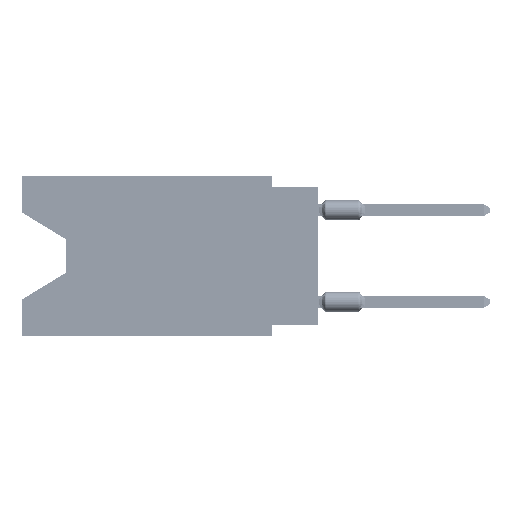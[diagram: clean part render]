
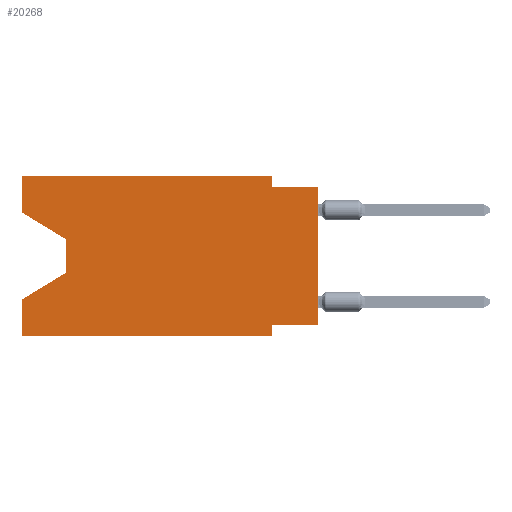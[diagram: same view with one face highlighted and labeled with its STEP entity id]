
A CAD part, left-side view. The second image highlights one B-rep face of the part: STEP entity #20268.
In plain terms, the highlighted planar face has unit normal (-1, 0, 0).
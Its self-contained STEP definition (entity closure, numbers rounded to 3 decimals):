
#35 = VECTOR ( 'NONE', #18206, 1000. ) ;
#1812 = ORIENTED_EDGE ( 'NONE', *, *, #26979, .F. ) ;
#2176 = LINE ( 'NONE', #37560, #27442 ) ;
#2943 = DIRECTION ( 'NONE',  ( 0., 1., 0. ) ) ;
#2965 = ORIENTED_EDGE ( 'NONE', *, *, #28584, .F. ) ;
#3649 = ORIENTED_EDGE ( 'NONE', *, *, #36116, .T. ) ;
#5922 = VERTEX_POINT ( 'NONE', #71807 ) ;
#6380 = VECTOR ( 'NONE', #44592, 1000. ) ;
#7038 = ORIENTED_EDGE ( 'NONE', *, *, #61734, .T. ) ;
#7966 = CARTESIAN_POINT ( 'NONE',  ( 0., 2.54, -8.89 ) ) ;
#8591 = CARTESIAN_POINT ( 'NONE',  ( 0., 16.383, 0. ) ) ;
#8744 = VERTEX_POINT ( 'NONE', #57537 ) ;
#9004 = EDGE_CURVE ( 'NONE', #44556, #27922, #29869, .T. ) ;
#9166 = DIRECTION ( 'NONE',  ( 0., -1., 0. ) ) ;
#9550 = LINE ( 'NONE', #32517, #25673 ) ;
#9578 = VERTEX_POINT ( 'NONE', #7966 ) ;
#12994 = LINE ( 'NONE', #37083, #18165 ) ;
#14210 = EDGE_CURVE ( 'NONE', #54224, #9578, #33137, .T. ) ;
#15890 = AXIS2_PLACEMENT_3D ( 'NONE', #19984, #43703, #32421 ) ;
#17105 = CARTESIAN_POINT ( 'NONE',  ( 0., 13.97, -3.505 ) ) ;
#18165 = VECTOR ( 'NONE', #60837, 1000. ) ;
#18206 = DIRECTION ( 'NONE',  ( 0., 0., 1. ) ) ;
#18877 = EDGE_CURVE ( 'NONE', #28221, #70979, #35831, .T. ) ;
#19884 = EDGE_CURVE ( 'NONE', #70979, #8744, #37947, .T. ) ;
#19984 = CARTESIAN_POINT ( 'NONE',  ( 0., 16.383, 0. ) ) ;
#20201 = EDGE_CURVE ( 'NONE', #27922, #28221, #35183, .T. ) ;
#20268 = ADVANCED_FACE ( 'NONE', ( #55393 ), #56157, .F. ) ;
#20823 = LINE ( 'NONE', #55856, #72713 ) ;
#23395 = VERTEX_POINT ( 'NONE', #60676 ) ;
#24446 = VECTOR ( 'NONE', #72033, 1000. ) ;
#24466 = DIRECTION ( 'NONE',  ( 0., 0.855, -0.519 ) ) ;
#24765 = CARTESIAN_POINT ( 'NONE',  ( 0., 2.54, 0. ) ) ;
#25241 = EDGE_LOOP ( 'NONE', ( #30478, #45612, #25558, #2965, #7038, #35270, #1812, #3649, #56038, #54397, #64348, #45249 ) ) ;
#25558 = ORIENTED_EDGE ( 'NONE', *, *, #73680, .T. ) ;
#25673 = VECTOR ( 'NONE', #57395, 1000. ) ;
#26979 = EDGE_CURVE ( 'NONE', #5922, #54224, #20823, .T. ) ;
#27442 = VECTOR ( 'NONE', #54706, 1000. ) ;
#27922 = VERTEX_POINT ( 'NONE', #8591 ) ;
#28221 = VERTEX_POINT ( 'NONE', #24765 ) ;
#28584 = EDGE_CURVE ( 'NONE', #55753, #42549, #12994, .T. ) ;
#29869 = LINE ( 'NONE', #36463, #35 ) ;
#30112 = CARTESIAN_POINT ( 'NONE',  ( 0., 16.383, -2.038 ) ) ;
#30478 = ORIENTED_EDGE ( 'NONE', *, *, #62757, .T. ) ;
#32421 = DIRECTION ( 'NONE',  ( 0., 0., -1. ) ) ;
#32517 = CARTESIAN_POINT ( 'NONE',  ( 0., 13.97, -3.505 ) ) ;
#33137 = LINE ( 'NONE', #56873, #39902 ) ;
#34991 = CARTESIAN_POINT ( 'NONE',  ( 0., 0., 0. ) ) ;
#35183 = LINE ( 'NONE', #53463, #54441 ) ;
#35270 = ORIENTED_EDGE ( 'NONE', *, *, #14210, .F. ) ;
#35279 = CARTESIAN_POINT ( 'NONE',  ( 0., 2.54, -8.255 ) ) ;
#35831 = LINE ( 'NONE', #48288, #24446 ) ;
#36116 = EDGE_CURVE ( 'NONE', #5922, #8744, #59117, .T. ) ;
#36463 = CARTESIAN_POINT ( 'NONE',  ( 0., 16.383, 0. ) ) ;
#37083 = CARTESIAN_POINT ( 'NONE',  ( 0., 16.383, 0. ) ) ;
#37560 = CARTESIAN_POINT ( 'NONE',  ( 0., 16.383, -8.89 ) ) ;
#37947 = LINE ( 'NONE', #72623, #64324 ) ;
#39902 = VECTOR ( 'NONE', #44432, 1000. ) ;
#41163 = VECTOR ( 'NONE', #71950, 1000. ) ;
#41974 = CARTESIAN_POINT ( 'NONE',  ( 0., 16.383, -6.852 ) ) ;
#42549 = VERTEX_POINT ( 'NONE', #41974 ) ;
#42808 = CARTESIAN_POINT ( 'NONE',  ( 0., 16.383, -8.89 ) ) ;
#43703 = DIRECTION ( 'NONE',  ( 1., 0., 0. ) ) ;
#43832 = LINE ( 'NONE', #67576, #6380 ) ;
#43899 = CARTESIAN_POINT ( 'NONE',  ( 0., 13.97, -5.385 ) ) ;
#44432 = DIRECTION ( 'NONE',  ( 0., 0., -1. ) ) ;
#44556 = VERTEX_POINT ( 'NONE', #30112 ) ;
#44592 = DIRECTION ( 'NONE',  ( 0., -0.855, -0.519 ) ) ;
#45249 = ORIENTED_EDGE ( 'NONE', *, *, #9004, .F. ) ;
#45612 = ORIENTED_EDGE ( 'NONE', *, *, #75224, .T. ) ;
#45865 = CARTESIAN_POINT ( 'NONE',  ( 0., 2.54, -0.635 ) ) ;
#46859 = DIRECTION ( 'NONE',  ( 0., -1., 0. ) ) ;
#48288 = CARTESIAN_POINT ( 'NONE',  ( 0., 2.54, 0. ) ) ;
#50524 = VECTOR ( 'NONE', #24466, 1000. ) ;
#53463 = CARTESIAN_POINT ( 'NONE',  ( 0., 16.383, 0. ) ) ;
#54034 = LINE ( 'NONE', #43899, #50524 ) ;
#54224 = VERTEX_POINT ( 'NONE', #35279 ) ;
#54397 = ORIENTED_EDGE ( 'NONE', *, *, #18877, .F. ) ;
#54441 = VECTOR ( 'NONE', #46859, 1000. ) ;
#54706 = DIRECTION ( 'NONE',  ( 0., -1., 0. ) ) ;
#55393 = FACE_OUTER_BOUND ( 'NONE', #25241, .T. ) ;
#55753 = VERTEX_POINT ( 'NONE', #42808 ) ;
#55856 = CARTESIAN_POINT ( 'NONE',  ( 0., 0., -8.255 ) ) ;
#56038 = ORIENTED_EDGE ( 'NONE', *, *, #19884, .F. ) ;
#56157 = PLANE ( 'NONE',  #15890 ) ;
#56873 = CARTESIAN_POINT ( 'NONE',  ( 0., 2.54, -8.89 ) ) ;
#57395 = DIRECTION ( 'NONE',  ( 0., 0., -1. ) ) ;
#57449 = VERTEX_POINT ( 'NONE', #17105 ) ;
#57537 = CARTESIAN_POINT ( 'NONE',  ( 0., 0., -0.635 ) ) ;
#59117 = LINE ( 'NONE', #34991, #41163 ) ;
#60676 = CARTESIAN_POINT ( 'NONE',  ( 0., 13.97, -5.385 ) ) ;
#60837 = DIRECTION ( 'NONE',  ( 0., 0., 1. ) ) ;
#61734 = EDGE_CURVE ( 'NONE', #55753, #9578, #2176, .T. ) ;
#62757 = EDGE_CURVE ( 'NONE', #44556, #57449, #43832, .T. ) ;
#64324 = VECTOR ( 'NONE', #9166, 1000. ) ;
#64348 = ORIENTED_EDGE ( 'NONE', *, *, #20201, .F. ) ;
#67576 = CARTESIAN_POINT ( 'NONE',  ( 0., 16.383, -2.038 ) ) ;
#70979 = VERTEX_POINT ( 'NONE', #45865 ) ;
#71807 = CARTESIAN_POINT ( 'NONE',  ( 0., 0., -8.255 ) ) ;
#71950 = DIRECTION ( 'NONE',  ( 0., 0., 1. ) ) ;
#72033 = DIRECTION ( 'NONE',  ( 0., 0., -1. ) ) ;
#72623 = CARTESIAN_POINT ( 'NONE',  ( 0., 0., -0.635 ) ) ;
#72713 = VECTOR ( 'NONE', #2943, 1000. ) ;
#73680 = EDGE_CURVE ( 'NONE', #23395, #42549, #54034, .T. ) ;
#75224 = EDGE_CURVE ( 'NONE', #57449, #23395, #9550, .T. ) ;
